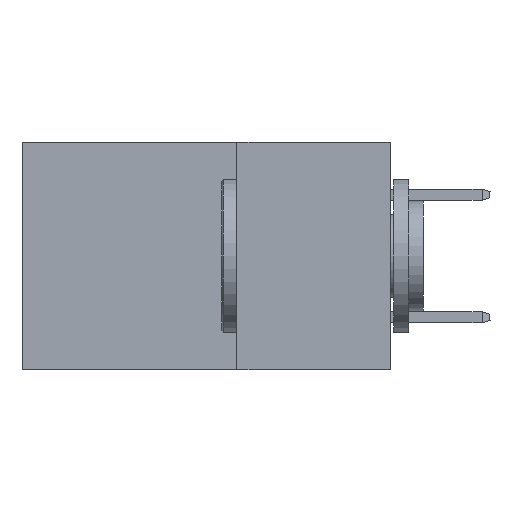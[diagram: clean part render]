
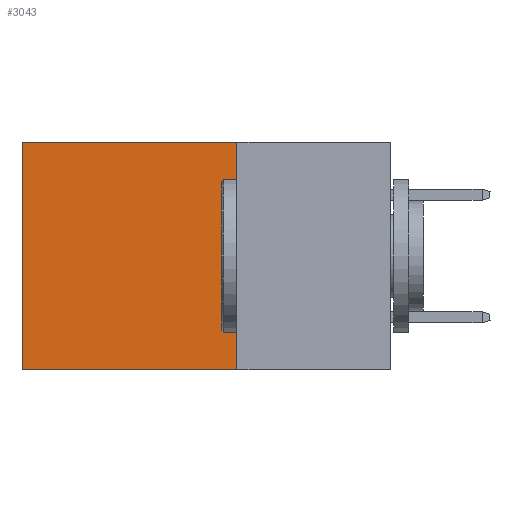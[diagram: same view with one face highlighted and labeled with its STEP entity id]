
A CAD part, left-side view. The second image highlights one B-rep face of the part: STEP entity #3043.
In plain terms, the highlighted planar face has unit normal (-1, 0, 0).
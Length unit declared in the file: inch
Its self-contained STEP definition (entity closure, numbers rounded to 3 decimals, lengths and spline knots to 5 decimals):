
#31 = CARTESIAN_POINT ( 'NONE',  ( 0.2875, 0.6, 0. ) ) ;
#113 = VECTOR ( 'NONE', #18226, 39.37008 ) ;
#738 = LINE ( 'NONE', #10959, #113 ) ;
#1470 = DIRECTION ( 'NONE',  ( 0., 0., -1. ) ) ;
#1952 = VERTEX_POINT ( 'NONE', #11396 ) ;
#3043 = ADVANCED_FACE ( 'NONE', ( #12421 ), #3060, .F. ) ;
#3060 = PLANE ( 'NONE',  #9821 ) ;
#3425 = VERTEX_POINT ( 'NONE', #19392 ) ;
#3648 = VECTOR ( 'NONE', #13198, 39.37008 ) ;
#4928 = ORIENTED_EDGE ( 'NONE', *, *, #23828, .T. ) ;
#5014 = ORIENTED_EDGE ( 'NONE', *, *, #16106, .F. ) ;
#5562 = CARTESIAN_POINT ( 'NONE',  ( 0.2875, 0.25, 0. ) ) ;
#6699 = CARTESIAN_POINT ( 'NONE',  ( 0.2875, 0.6, 0. ) ) ;
#7059 = EDGE_CURVE ( 'NONE', #3425, #16434, #738, .T. ) ;
#7875 = DIRECTION ( 'NONE',  ( 1., 0., 0. ) ) ;
#8587 = LINE ( 'NONE', #31, #3648 ) ;
#9486 = VERTEX_POINT ( 'NONE', #6699 ) ;
#9821 = AXIS2_PLACEMENT_3D ( 'NONE', #5562, #7875, #1470 ) ;
#10959 = CARTESIAN_POINT ( 'NONE',  ( 0.2875, 0.25, -0.37 ) ) ;
#11200 = ORIENTED_EDGE ( 'NONE', *, *, #17240, .T. ) ;
#11396 = CARTESIAN_POINT ( 'NONE',  ( 0.2875, 0.25, 0. ) ) ;
#11667 = CARTESIAN_POINT ( 'NONE',  ( 0.2875, 0.25, 0. ) ) ;
#12421 = FACE_OUTER_BOUND ( 'NONE', #17098, .T. ) ;
#12560 = VECTOR ( 'NONE', #13497, 39.37008 ) ;
#13198 = DIRECTION ( 'NONE',  ( 0., 0., -1. ) ) ;
#13497 = DIRECTION ( 'NONE',  ( 0., 1., 0. ) ) ;
#13674 = LINE ( 'NONE', #11667, #12560 ) ;
#13775 = CARTESIAN_POINT ( 'NONE',  ( 0.2875, 0.25, 0. ) ) ;
#15433 = ORIENTED_EDGE ( 'NONE', *, *, #7059, .F. ) ;
#15576 = DIRECTION ( 'NONE',  ( 0., 0., -1. ) ) ;
#16106 = EDGE_CURVE ( 'NONE', #1952, #3425, #21612, .T. ) ;
#16434 = VERTEX_POINT ( 'NONE', #23584 ) ;
#17098 = EDGE_LOOP ( 'NONE', ( #4928, #15433, #5014, #11200 ) ) ;
#17112 = VECTOR ( 'NONE', #15576, 39.37008 ) ;
#17240 = EDGE_CURVE ( 'NONE', #1952, #9486, #13674, .T. ) ;
#18226 = DIRECTION ( 'NONE',  ( 0., 1., 0. ) ) ;
#19392 = CARTESIAN_POINT ( 'NONE',  ( 0.2875, 0.25, -0.37 ) ) ;
#21612 = LINE ( 'NONE', #13775, #17112 ) ;
#23584 = CARTESIAN_POINT ( 'NONE',  ( 0.2875, 0.6, -0.37 ) ) ;
#23828 = EDGE_CURVE ( 'NONE', #9486, #16434, #8587, .T. ) ;
